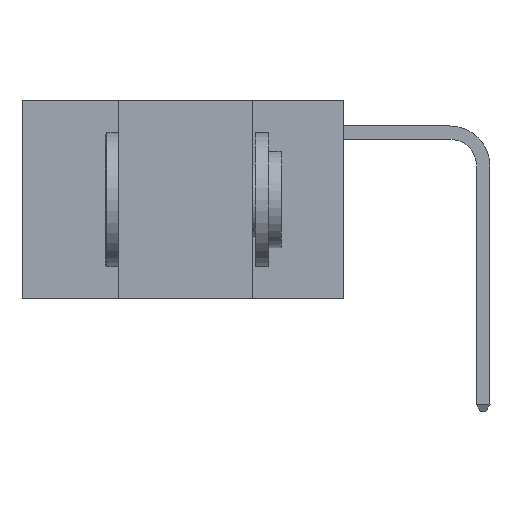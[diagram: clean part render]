
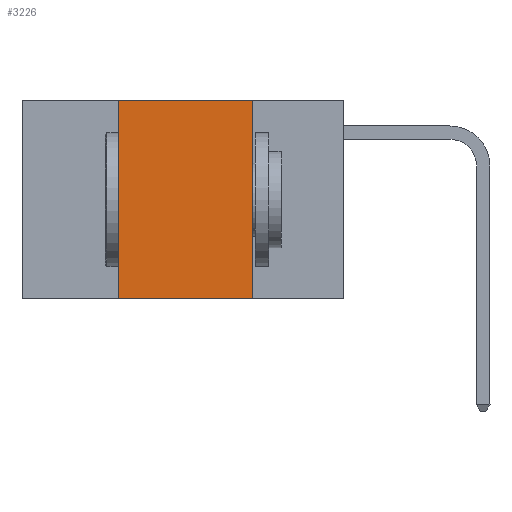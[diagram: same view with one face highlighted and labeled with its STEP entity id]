
A CAD part, left-side view. The second image highlights one B-rep face of the part: STEP entity #3226.
In plain terms, the highlighted planar face has unit normal (-1, 0, 0).
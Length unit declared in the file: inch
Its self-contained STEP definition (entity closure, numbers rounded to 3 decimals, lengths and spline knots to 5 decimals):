
#24 = ORIENTED_EDGE ( 'NONE', *, *, #9313, .T. ) ;
#472 = VECTOR ( 'NONE', #6186, 39.37008 ) ;
#1118 = VERTEX_POINT ( 'NONE', #3559 ) ;
#1212 = VECTOR ( 'NONE', #5051, 39.37008 ) ;
#1222 = PLANE ( 'NONE',  #2260 ) ;
#1835 = VERTEX_POINT ( 'NONE', #4050 ) ;
#2031 = DIRECTION ( 'NONE',  ( 0., 0., -1. ) ) ;
#2260 = AXIS2_PLACEMENT_3D ( 'NONE', #7881, #4911, #2031 ) ;
#2465 = LINE ( 'NONE', #3892, #3987 ) ;
#2848 = CARTESIAN_POINT ( 'NONE',  ( 0., 0.17, 0. ) ) ;
#3075 = ORIENTED_EDGE ( 'NONE', *, *, #6044, .F. ) ;
#3151 = VERTEX_POINT ( 'NONE', #4273 ) ;
#3181 = DIRECTION ( 'NONE',  ( 0., 0., 1. ) ) ;
#3226 = ADVANCED_FACE ( 'NONE', ( #6312 ), #1222, .F. ) ;
#3559 = CARTESIAN_POINT ( 'NONE',  ( 0., 0.17, -0.37 ) ) ;
#3892 = CARTESIAN_POINT ( 'NONE',  ( 0., 0.42, 0. ) ) ;
#3987 = VECTOR ( 'NONE', #3181, 39.37008 ) ;
#4050 = CARTESIAN_POINT ( 'NONE',  ( 0., 0.42, 0. ) ) ;
#4273 = CARTESIAN_POINT ( 'NONE',  ( 0., 0.42, -0.37 ) ) ;
#4371 = ORIENTED_EDGE ( 'NONE', *, *, #5262, .F. ) ;
#4911 = DIRECTION ( 'NONE',  ( 1., 0., 0. ) ) ;
#5051 = DIRECTION ( 'NONE',  ( 0., 0., -1. ) ) ;
#5262 = EDGE_CURVE ( 'NONE', #9250, #1118, #9321, .T. ) ;
#5345 = CARTESIAN_POINT ( 'NONE',  ( 0., 0.6, -0.37 ) ) ;
#6044 = EDGE_CURVE ( 'NONE', #1835, #9250, #6286, .T. ) ;
#6100 = LINE ( 'NONE', #5345, #8065 ) ;
#6186 = DIRECTION ( 'NONE',  ( 0., -1., 0. ) ) ;
#6286 = LINE ( 'NONE', #9239, #472 ) ;
#6312 = FACE_OUTER_BOUND ( 'NONE', #8270, .T. ) ;
#6610 = CARTESIAN_POINT ( 'NONE',  ( 0., 0.17, 0. ) ) ;
#6728 = EDGE_CURVE ( 'NONE', #3151, #1835, #2465, .T. ) ;
#6770 = ORIENTED_EDGE ( 'NONE', *, *, #6728, .F. ) ;
#7481 = DIRECTION ( 'NONE',  ( 0., -1., 0. ) ) ;
#7881 = CARTESIAN_POINT ( 'NONE',  ( 0., 0.6, 0. ) ) ;
#8065 = VECTOR ( 'NONE', #7481, 39.37008 ) ;
#8270 = EDGE_LOOP ( 'NONE', ( #4371, #3075, #6770, #24 ) ) ;
#9239 = CARTESIAN_POINT ( 'NONE',  ( 0., 0.6, 0. ) ) ;
#9250 = VERTEX_POINT ( 'NONE', #6610 ) ;
#9313 = EDGE_CURVE ( 'NONE', #3151, #1118, #6100, .T. ) ;
#9321 = LINE ( 'NONE', #2848, #1212 ) ;
